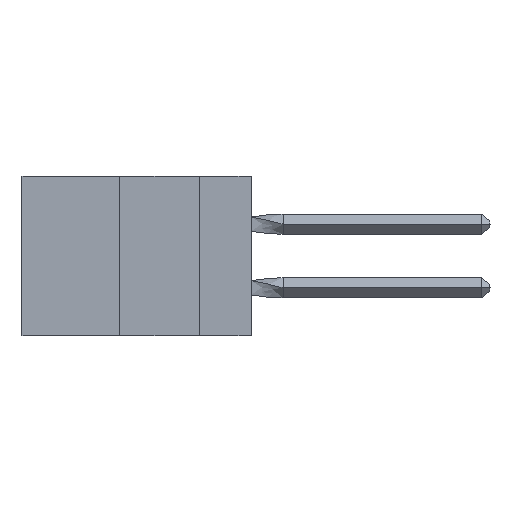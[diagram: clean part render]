
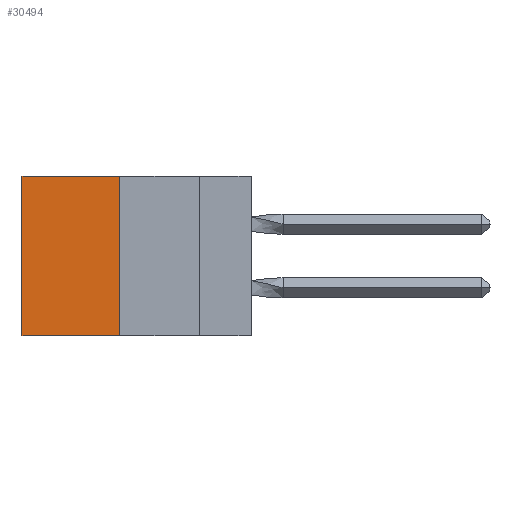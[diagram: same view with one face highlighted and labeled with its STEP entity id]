
A CAD part, left-side view. The second image highlights one B-rep face of the part: STEP entity #30494.
In plain terms, the highlighted planar face has unit normal (-1, 0, 0).
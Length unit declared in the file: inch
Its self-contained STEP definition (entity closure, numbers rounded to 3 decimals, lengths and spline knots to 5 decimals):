
#638 = CARTESIAN_POINT ( 'NONE',  ( 0.305, 0.413, -0.5 ) ) ;
#1138 = CARTESIAN_POINT ( 'NONE',  ( 0.305, 0.413, 0. ) ) ;
#3845 = EDGE_CURVE ( 'NONE', #22235, #32095, #35803, .T. ) ;
#4301 = DIRECTION ( 'NONE',  ( 0., 1., 0. ) ) ;
#4780 = EDGE_CURVE ( 'NONE', #40116, #32095, #26870, .T. ) ;
#5852 = VECTOR ( 'NONE', #10125, 39.37008 ) ;
#9333 = DIRECTION ( 'NONE',  ( 0., 0., -1. ) ) ;
#9420 = LINE ( 'NONE', #23872, #42129 ) ;
#10125 = DIRECTION ( 'NONE',  ( 0., 0., -1. ) ) ;
#12312 = VECTOR ( 'NONE', #34579, 39.37008 ) ;
#12721 = ORIENTED_EDGE ( 'NONE', *, *, #4780, .F. ) ;
#14449 = EDGE_CURVE ( 'NONE', #20779, #22235, #9420, .T. ) ;
#14538 = ORIENTED_EDGE ( 'NONE', *, *, #40895, .F. ) ;
#15121 = CARTESIAN_POINT ( 'NONE',  ( 0.305, 0.72, 0. ) ) ;
#15825 = CARTESIAN_POINT ( 'NONE',  ( 0.305, 0.413, -0.5 ) ) ;
#20346 = AXIS2_PLACEMENT_3D ( 'NONE', #638, #36629, #9333 ) ;
#20779 = VERTEX_POINT ( 'NONE', #1138 ) ;
#22235 = VERTEX_POINT ( 'NONE', #15121 ) ;
#22449 = CARTESIAN_POINT ( 'NONE',  ( 0.305, 0.413, -0.5 ) ) ;
#23230 = PLANE ( 'NONE',  #20346 ) ;
#23872 = CARTESIAN_POINT ( 'NONE',  ( 0.305, 0.413, 0. ) ) ;
#26870 = LINE ( 'NONE', #32264, #33522 ) ;
#27555 = CARTESIAN_POINT ( 'NONE',  ( 0.305, 0.72, -0.5 ) ) ;
#30494 = ADVANCED_FACE ( 'NONE', ( #32232 ), #23230, .F. ) ;
#31472 = ORIENTED_EDGE ( 'NONE', *, *, #14449, .T. ) ;
#32095 = VERTEX_POINT ( 'NONE', #27555 ) ;
#32232 = FACE_OUTER_BOUND ( 'NONE', #37352, .T. ) ;
#32264 = CARTESIAN_POINT ( 'NONE',  ( 0.305, 0.413, -0.5 ) ) ;
#33522 = VECTOR ( 'NONE', #41407, 39.37008 ) ;
#34579 = DIRECTION ( 'NONE',  ( 0., 0., -1. ) ) ;
#35803 = LINE ( 'NONE', #37595, #12312 ) ;
#36629 = DIRECTION ( 'NONE',  ( 1., 0., 0. ) ) ;
#37352 = EDGE_LOOP ( 'NONE', ( #39999, #12721, #14538, #31472 ) ) ;
#37595 = CARTESIAN_POINT ( 'NONE',  ( 0.305, 0.72, -0.5 ) ) ;
#39999 = ORIENTED_EDGE ( 'NONE', *, *, #3845, .T. ) ;
#40116 = VERTEX_POINT ( 'NONE', #15825 ) ;
#40631 = LINE ( 'NONE', #22449, #5852 ) ;
#40895 = EDGE_CURVE ( 'NONE', #20779, #40116, #40631, .T. ) ;
#41407 = DIRECTION ( 'NONE',  ( 0., 1., 0. ) ) ;
#42129 = VECTOR ( 'NONE', #4301, 39.37008 ) ;
